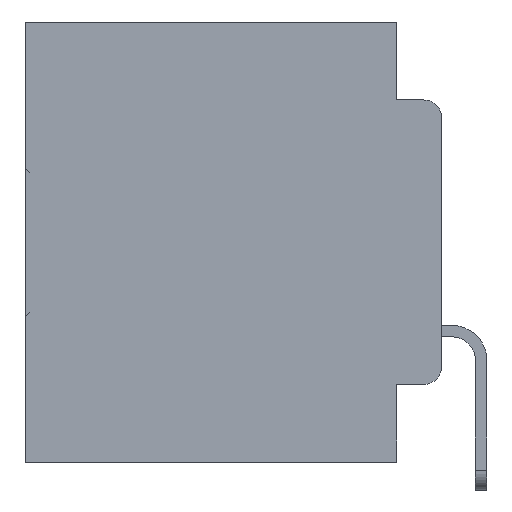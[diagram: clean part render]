
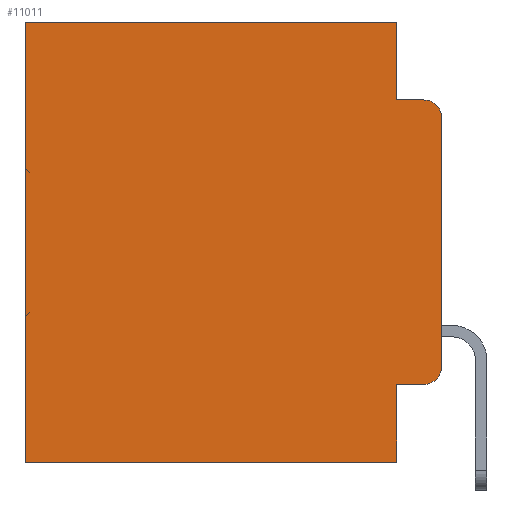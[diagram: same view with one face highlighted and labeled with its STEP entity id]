
A CAD part, left-side view. The second image highlights one B-rep face of the part: STEP entity #11011.
In plain terms, the highlighted planar face has unit normal (-1, 0, 0).
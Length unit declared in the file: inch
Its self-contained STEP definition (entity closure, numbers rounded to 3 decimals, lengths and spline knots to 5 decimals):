
#77 = ORIENTED_EDGE ( 'NONE', *, *, #18107, .T. ) ;
#136 = VECTOR ( 'NONE', #19372, 39.37008 ) ;
#762 = VECTOR ( 'NONE', #33084, 39.37008 ) ;
#1223 = CARTESIAN_POINT ( 'NONE',  ( 0.298, 0.473, -0.5 ) ) ;
#1352 = AXIS2_PLACEMENT_3D ( 'NONE', #24630, #9456, #27111 ) ;
#1755 = EDGE_CURVE ( 'NONE', #11854, #20219, #29128, .T. ) ;
#1876 = VERTEX_POINT ( 'NONE', #29196 ) ;
#2050 = LINE ( 'NONE', #25206, #762 ) ;
#2378 = ORIENTED_EDGE ( 'NONE', *, *, #1755, .F. ) ;
#2722 = ORIENTED_EDGE ( 'NONE', *, *, #5768, .T. ) ;
#2817 = VECTOR ( 'NONE', #8789, 39.37008 ) ;
#4117 = DIRECTION ( 'NONE',  ( 0., 1., 0. ) ) ;
#4277 = ORIENTED_EDGE ( 'NONE', *, *, #11234, .F. ) ;
#4528 = DIRECTION ( 'NONE',  ( 1., 0., 0. ) ) ;
#4720 = CIRCLE ( 'NONE', #20847, 0.02 ) ;
#4838 = VECTOR ( 'NONE', #16870, 39.37008 ) ;
#5273 = AXIS2_PLACEMENT_3D ( 'NONE', #7172, #4528, #22682 ) ;
#5768 = EDGE_CURVE ( 'NONE', #1876, #31871, #4720, .T. ) ;
#7172 = CARTESIAN_POINT ( 'NONE',  ( 0.298, 0., 0. ) ) ;
#7289 = EDGE_CURVE ( 'NONE', #24647, #33137, #24978, .T. ) ;
#7385 = CARTESIAN_POINT ( 'NONE',  ( 0.298, 0., -0.1085 ) ) ;
#7528 = DIRECTION ( 'NONE',  ( -1., 0., 0. ) ) ;
#7554 = CARTESIAN_POINT ( 'NONE',  ( 0.298, 0., -0.3915 ) ) ;
#7658 = LINE ( 'NONE', #19153, #136 ) ;
#8789 = DIRECTION ( 'NONE',  ( 0., 0., -1. ) ) ;
#9209 = CARTESIAN_POINT ( 'NONE',  ( 0.298, 0., -0.5 ) ) ;
#9417 = EDGE_CURVE ( 'NONE', #19732, #1876, #23934, .T. ) ;
#9456 = DIRECTION ( 'NONE',  ( -1., 0., 0. ) ) ;
#10162 = LINE ( 'NONE', #19084, #2817 ) ;
#10847 = CARTESIAN_POINT ( 'NONE',  ( 0.298, 0.051, 0. ) ) ;
#11011 = ADVANCED_FACE ( 'NONE', ( #24543 ), #20221, .F. ) ;
#11119 = ORIENTED_EDGE ( 'NONE', *, *, #9417, .T. ) ;
#11234 = EDGE_CURVE ( 'NONE', #19732, #11854, #23404, .T. ) ;
#11854 = VERTEX_POINT ( 'NONE', #20607 ) ;
#12661 = CARTESIAN_POINT ( 'NONE',  ( 0.298, 0.051, -0.4115 ) ) ;
#13161 = ORIENTED_EDGE ( 'NONE', *, *, #32944, .F. ) ;
#13413 = CARTESIAN_POINT ( 'NONE',  ( 0.298, 0.051, -0.4115 ) ) ;
#14714 = CARTESIAN_POINT ( 'NONE',  ( 0.298, 0.02, -0.0885 ) ) ;
#16870 = DIRECTION ( 'NONE',  ( 0., 0., -1. ) ) ;
#17301 = VECTOR ( 'NONE', #23555, 39.37008 ) ;
#18107 = EDGE_CURVE ( 'NONE', #33137, #20219, #26144, .T. ) ;
#18436 = VECTOR ( 'NONE', #4117, 39.37008 ) ;
#18478 = ORIENTED_EDGE ( 'NONE', *, *, #21425, .F. ) ;
#18873 = EDGE_LOOP ( 'NONE', ( #13161, #25396, #18478, #25201, #30258, #77, #2378, #4277, #11119, #2722 ) ) ;
#18962 = CARTESIAN_POINT ( 'NONE',  ( 0.298, 0.473, 0. ) ) ;
#19084 = CARTESIAN_POINT ( 'NONE',  ( 0.298, 0., 0. ) ) ;
#19153 = CARTESIAN_POINT ( 'NONE',  ( 0.298, 0.051, -0.0885 ) ) ;
#19372 = DIRECTION ( 'NONE',  ( 0., -1., 0. ) ) ;
#19732 = VERTEX_POINT ( 'NONE', #12661 ) ;
#19791 = EDGE_CURVE ( 'NONE', #24647, #32347, #2050, .T. ) ;
#20219 = VERTEX_POINT ( 'NONE', #1223 ) ;
#20221 = PLANE ( 'NONE',  #5273 ) ;
#20607 = CARTESIAN_POINT ( 'NONE',  ( 0.298, 0.051, -0.5 ) ) ;
#20847 = AXIS2_PLACEMENT_3D ( 'NONE', #22881, #7528, #25337 ) ;
#21425 = EDGE_CURVE ( 'NONE', #32347, #22481, #7658, .T. ) ;
#21832 = DIRECTION ( 'NONE',  ( 0., 1., 0. ) ) ;
#22481 = VERTEX_POINT ( 'NONE', #14714 ) ;
#22581 = VECTOR ( 'NONE', #21832, 39.37008 ) ;
#22682 = DIRECTION ( 'NONE',  ( 0., 0., -1. ) ) ;
#22881 = CARTESIAN_POINT ( 'NONE',  ( 0.298, 0.02, -0.3915 ) ) ;
#23378 = CARTESIAN_POINT ( 'NONE',  ( 0.298, 0.473, 0. ) ) ;
#23404 = LINE ( 'NONE', #10847, #29162 ) ;
#23555 = DIRECTION ( 'NONE',  ( 0., -1., 0. ) ) ;
#23934 = LINE ( 'NONE', #13413, #17301 ) ;
#24543 = FACE_OUTER_BOUND ( 'NONE', #18873, .T. ) ;
#24575 = CARTESIAN_POINT ( 'NONE',  ( 0.298, 0.051, -0.0885 ) ) ;
#24630 = CARTESIAN_POINT ( 'NONE',  ( 0.298, 0.02, -0.1085 ) ) ;
#24647 = VERTEX_POINT ( 'NONE', #25521 ) ;
#24978 = LINE ( 'NONE', #27152, #18436 ) ;
#25201 = ORIENTED_EDGE ( 'NONE', *, *, #19791, .F. ) ;
#25206 = CARTESIAN_POINT ( 'NONE',  ( 0.298, 0.051, 0. ) ) ;
#25247 = CIRCLE ( 'NONE', #1352, 0.02 ) ;
#25337 = DIRECTION ( 'NONE',  ( 0., 0., -1. ) ) ;
#25396 = ORIENTED_EDGE ( 'NONE', *, *, #28026, .T. ) ;
#25521 = CARTESIAN_POINT ( 'NONE',  ( 0.298, 0.051, 0. ) ) ;
#26144 = LINE ( 'NONE', #23378, #4838 ) ;
#27111 = DIRECTION ( 'NONE',  ( 0., 0., -1. ) ) ;
#27152 = CARTESIAN_POINT ( 'NONE',  ( 0.298, 0., 0. ) ) ;
#28026 = EDGE_CURVE ( 'NONE', #32527, #22481, #25247, .T. ) ;
#29128 = LINE ( 'NONE', #9209, #22581 ) ;
#29162 = VECTOR ( 'NONE', #33294, 39.37008 ) ;
#29196 = CARTESIAN_POINT ( 'NONE',  ( 0.298, 0.02, -0.4115 ) ) ;
#30258 = ORIENTED_EDGE ( 'NONE', *, *, #7289, .T. ) ;
#31871 = VERTEX_POINT ( 'NONE', #7554 ) ;
#32347 = VERTEX_POINT ( 'NONE', #24575 ) ;
#32527 = VERTEX_POINT ( 'NONE', #7385 ) ;
#32944 = EDGE_CURVE ( 'NONE', #32527, #31871, #10162, .T. ) ;
#33084 = DIRECTION ( 'NONE',  ( 0., 0., -1. ) ) ;
#33137 = VERTEX_POINT ( 'NONE', #18962 ) ;
#33294 = DIRECTION ( 'NONE',  ( 0., 0., -1. ) ) ;
